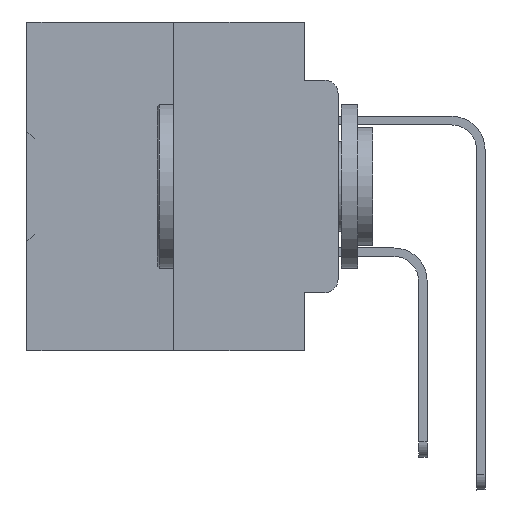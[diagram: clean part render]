
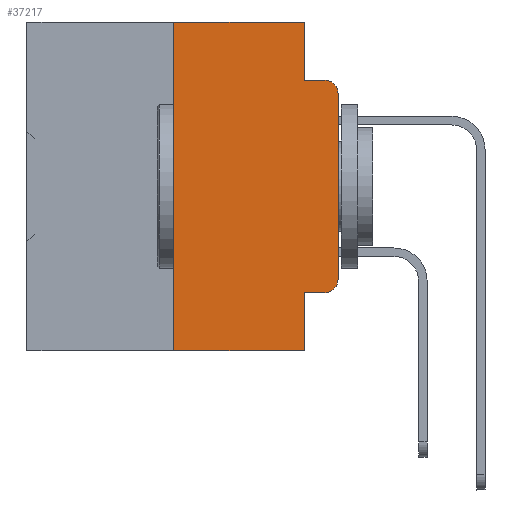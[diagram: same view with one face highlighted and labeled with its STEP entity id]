
A CAD part, left-side view. The second image highlights one B-rep face of the part: STEP entity #37217.
In plain terms, the highlighted planar face has unit normal (-1, 0, 0).
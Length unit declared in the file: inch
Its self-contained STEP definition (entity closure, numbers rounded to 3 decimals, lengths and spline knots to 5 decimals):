
#593 = DIRECTION ( 'NONE',  ( -1., 0., 0. ) ) ;
#777 = ORIENTED_EDGE ( 'NONE', *, *, #33420, .T. ) ;
#889 = LINE ( 'NONE', #29348, #17146 ) ;
#1034 = CARTESIAN_POINT ( 'NONE',  ( 0., 0.473, 0. ) ) ;
#1431 = CARTESIAN_POINT ( 'NONE',  ( 0., 0., 0. ) ) ;
#2792 = EDGE_CURVE ( 'NONE', #37933, #30519, #3494, .T. ) ;
#3290 = CARTESIAN_POINT ( 'NONE',  ( 0., 0.02, -0.3915 ) ) ;
#3494 = LINE ( 'NONE', #14546, #27189 ) ;
#3886 = CARTESIAN_POINT ( 'NONE',  ( 0., 0.051, 0. ) ) ;
#3997 = ORIENTED_EDGE ( 'NONE', *, *, #16350, .F. ) ;
#4343 = DIRECTION ( 'NONE',  ( 0., 0., -1. ) ) ;
#4499 = AXIS2_PLACEMENT_3D ( 'NONE', #3290, #25855, #6610 ) ;
#5541 = EDGE_CURVE ( 'NONE', #32332, #19436, #29896, .T. ) ;
#5704 = CARTESIAN_POINT ( 'NONE',  ( 0., 0.02, -0.4115 ) ) ;
#6556 = LINE ( 'NONE', #1431, #30093 ) ;
#6588 = ORIENTED_EDGE ( 'NONE', *, *, #9908, .F. ) ;
#6610 = DIRECTION ( 'NONE',  ( 0., 0., -1. ) ) ;
#7168 = LINE ( 'NONE', #12938, #15276 ) ;
#7265 = ORIENTED_EDGE ( 'NONE', *, *, #20649, .F. ) ;
#7738 = EDGE_CURVE ( 'NONE', #37816, #32332, #38970, .T. ) ;
#9908 = EDGE_CURVE ( 'NONE', #37816, #10576, #35885, .T. ) ;
#10447 = CARTESIAN_POINT ( 'NONE',  ( 0., 0.02, -0.0885 ) ) ;
#10576 = VERTEX_POINT ( 'NONE', #14691 ) ;
#11746 = CARTESIAN_POINT ( 'NONE',  ( 0., 0.051, 0. ) ) ;
#12135 = ORIENTED_EDGE ( 'NONE', *, *, #18489, .F. ) ;
#12195 = VERTEX_POINT ( 'NONE', #13460 ) ;
#12938 = CARTESIAN_POINT ( 'NONE',  ( 0., 0.051, -0.0885 ) ) ;
#13460 = CARTESIAN_POINT ( 'NONE',  ( 0., 0.051, -0.0885 ) ) ;
#14546 = CARTESIAN_POINT ( 'NONE',  ( 0., 0.473, 0. ) ) ;
#14691 = CARTESIAN_POINT ( 'NONE',  ( 0., 0.051, -0.5 ) ) ;
#15276 = VECTOR ( 'NONE', #16149, 39.37008 ) ;
#16149 = DIRECTION ( 'NONE',  ( 0., -1., 0. ) ) ;
#16350 = EDGE_CURVE ( 'NONE', #18035, #37933, #889, .T. ) ;
#17146 = VECTOR ( 'NONE', #32521, 39.37008 ) ;
#17191 = ORIENTED_EDGE ( 'NONE', *, *, #7738, .T. ) ;
#18035 = VERTEX_POINT ( 'NONE', #31723 ) ;
#18489 = EDGE_CURVE ( 'NONE', #30519, #12195, #32953, .T. ) ;
#18572 = AXIS2_PLACEMENT_3D ( 'NONE', #19985, #593, #23227 ) ;
#19436 = VERTEX_POINT ( 'NONE', #22540 ) ;
#19985 = CARTESIAN_POINT ( 'NONE',  ( 0., 0.02, -0.1085 ) ) ;
#20369 = FACE_OUTER_BOUND ( 'NONE', #36185, .T. ) ;
#20636 = ORIENTED_EDGE ( 'NONE', *, *, #2792, .F. ) ;
#20649 = EDGE_CURVE ( 'NONE', #12195, #22054, #7168, .T. ) ;
#20680 = ORIENTED_EDGE ( 'NONE', *, *, #31847, .T. ) ;
#22054 = VERTEX_POINT ( 'NONE', #10447 ) ;
#22540 = CARTESIAN_POINT ( 'NONE',  ( 0., 0., -0.3915 ) ) ;
#23227 = DIRECTION ( 'NONE',  ( 0., 0., -1. ) ) ;
#23535 = PLANE ( 'NONE',  #29700 ) ;
#23686 = DIRECTION ( 'NONE',  ( 1., 0., 0. ) ) ;
#24060 = DIRECTION ( 'NONE',  ( 0., 0., 1. ) ) ;
#24282 = ORIENTED_EDGE ( 'NONE', *, *, #5541, .T. ) ;
#25855 = DIRECTION ( 'NONE',  ( -1., 0., 0. ) ) ;
#26417 = LINE ( 'NONE', #32047, #41146 ) ;
#27189 = VECTOR ( 'NONE', #32446, 39.37008 ) ;
#27443 = CIRCLE ( 'NONE', #18572, 0.02 ) ;
#27527 = VECTOR ( 'NONE', #35908, 39.37008 ) ;
#28238 = DIRECTION ( 'NONE',  ( 0., -1., 0. ) ) ;
#29003 = DIRECTION ( 'NONE',  ( 0., -1., 0. ) ) ;
#29348 = CARTESIAN_POINT ( 'NONE',  ( 0., 0.25, 0. ) ) ;
#29700 = AXIS2_PLACEMENT_3D ( 'NONE', #1034, #23686, #4343 ) ;
#29711 = CARTESIAN_POINT ( 'NONE',  ( 0., 0.051, -0.4115 ) ) ;
#29896 = CIRCLE ( 'NONE', #4499, 0.02 ) ;
#30093 = VECTOR ( 'NONE', #24060, 39.37008 ) ;
#30519 = VERTEX_POINT ( 'NONE', #33203 ) ;
#30523 = CARTESIAN_POINT ( 'NONE',  ( 0., 0.25, 0. ) ) ;
#30595 = VECTOR ( 'NONE', #28238, 39.37008 ) ;
#30841 = DIRECTION ( 'NONE',  ( 0., 0., -1. ) ) ;
#31310 = EDGE_CURVE ( 'NONE', #33339, #22054, #27443, .T. ) ;
#31723 = CARTESIAN_POINT ( 'NONE',  ( 0., 0.25, -0.5 ) ) ;
#31847 = EDGE_CURVE ( 'NONE', #18035, #10576, #26417, .T. ) ;
#31961 = VECTOR ( 'NONE', #30841, 39.37008 ) ;
#32047 = CARTESIAN_POINT ( 'NONE',  ( 0., 0.473, -0.5 ) ) ;
#32332 = VERTEX_POINT ( 'NONE', #5704 ) ;
#32446 = DIRECTION ( 'NONE',  ( 0., -1., 0. ) ) ;
#32521 = DIRECTION ( 'NONE',  ( 0., 0., 1. ) ) ;
#32953 = LINE ( 'NONE', #11746, #31961 ) ;
#33203 = CARTESIAN_POINT ( 'NONE',  ( 0., 0.051, 0. ) ) ;
#33339 = VERTEX_POINT ( 'NONE', #39352 ) ;
#33420 = EDGE_CURVE ( 'NONE', #19436, #33339, #6556, .T. ) ;
#34414 = CARTESIAN_POINT ( 'NONE',  ( 0., 0.051, -0.4115 ) ) ;
#35311 = ORIENTED_EDGE ( 'NONE', *, *, #31310, .T. ) ;
#35885 = LINE ( 'NONE', #3886, #27527 ) ;
#35908 = DIRECTION ( 'NONE',  ( 0., 0., -1. ) ) ;
#36185 = EDGE_LOOP ( 'NONE', ( #777, #35311, #7265, #12135, #20636, #3997, #20680, #6588, #17191, #24282 ) ) ;
#37217 = ADVANCED_FACE ( 'NONE', ( #20369 ), #23535, .F. ) ;
#37816 = VERTEX_POINT ( 'NONE', #29711 ) ;
#37933 = VERTEX_POINT ( 'NONE', #30523 ) ;
#38970 = LINE ( 'NONE', #34414, #30595 ) ;
#39352 = CARTESIAN_POINT ( 'NONE',  ( 0., 0., -0.1085 ) ) ;
#41146 = VECTOR ( 'NONE', #29003, 39.37008 ) ;
